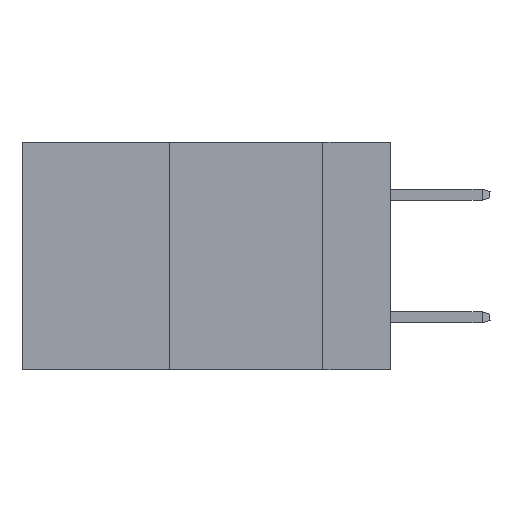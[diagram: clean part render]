
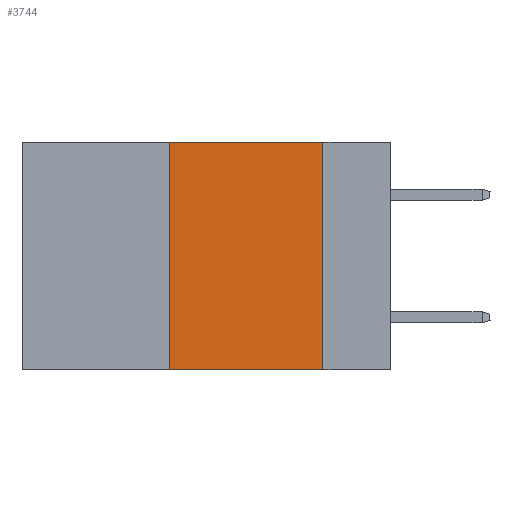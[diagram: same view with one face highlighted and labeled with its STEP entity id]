
A CAD part, left-side view. The second image highlights one B-rep face of the part: STEP entity #3744.
In plain terms, the highlighted planar face has unit normal (-1, 0, 0).
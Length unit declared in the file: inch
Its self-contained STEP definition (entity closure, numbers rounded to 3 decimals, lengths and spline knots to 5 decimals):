
#955 = CARTESIAN_POINT ( 'NONE',  ( 0., 0.11, 0. ) ) ;
#1171 = ORIENTED_EDGE ( 'NONE', *, *, #2881, .F. ) ;
#1340 = LINE ( 'NONE', #955, #3835 ) ;
#1670 = VERTEX_POINT ( 'NONE', #9632 ) ;
#1900 = ORIENTED_EDGE ( 'NONE', *, *, #5287, .T. ) ;
#2050 = VERTEX_POINT ( 'NONE', #5353 ) ;
#2430 = AXIS2_PLACEMENT_3D ( 'NONE', #10593, #5706, #5643 ) ;
#2775 = VERTEX_POINT ( 'NONE', #6938 ) ;
#2881 = EDGE_CURVE ( 'NONE', #2775, #2050, #11167, .T. ) ;
#3100 = DIRECTION ( 'NONE',  ( 0., 0., -1. ) ) ;
#3429 = ORIENTED_EDGE ( 'NONE', *, *, #8253, .F. ) ;
#3744 = ADVANCED_FACE ( 'NONE', ( #4328 ), #6311, .F. ) ;
#3835 = VECTOR ( 'NONE', #3100, 39.37008 ) ;
#4328 = FACE_OUTER_BOUND ( 'NONE', #7788, .T. ) ;
#5287 = EDGE_CURVE ( 'NONE', #2775, #1670, #8871, .T. ) ;
#5353 = CARTESIAN_POINT ( 'NONE',  ( 0., 0.36, 0. ) ) ;
#5643 = DIRECTION ( 'NONE',  ( 0., 0., -1. ) ) ;
#5706 = DIRECTION ( 'NONE',  ( 1., 0., 0. ) ) ;
#5998 = DIRECTION ( 'NONE',  ( 0., 0., 1. ) ) ;
#6028 = CARTESIAN_POINT ( 'NONE',  ( 0., 0.36, 0. ) ) ;
#6311 = PLANE ( 'NONE',  #2430 ) ;
#6621 = CARTESIAN_POINT ( 'NONE',  ( 0., 0.6, -0.37 ) ) ;
#6807 = EDGE_CURVE ( 'NONE', #9987, #1670, #1340, .T. ) ;
#6938 = CARTESIAN_POINT ( 'NONE',  ( 0., 0.36, -0.37 ) ) ;
#7747 = ORIENTED_EDGE ( 'NONE', *, *, #6807, .F. ) ;
#7788 = EDGE_LOOP ( 'NONE', ( #7747, #3429, #1171, #1900 ) ) ;
#8253 = EDGE_CURVE ( 'NONE', #2050, #9987, #12734, .T. ) ;
#8274 = VECTOR ( 'NONE', #12370, 39.37008 ) ;
#8312 = VECTOR ( 'NONE', #5998, 39.37008 ) ;
#8687 = CARTESIAN_POINT ( 'NONE',  ( 0., 0.11, 0. ) ) ;
#8871 = LINE ( 'NONE', #6621, #8274 ) ;
#9509 = CARTESIAN_POINT ( 'NONE',  ( 0., 0.6, 0. ) ) ;
#9553 = DIRECTION ( 'NONE',  ( 0., -1., 0. ) ) ;
#9632 = CARTESIAN_POINT ( 'NONE',  ( 0., 0.11, -0.37 ) ) ;
#9987 = VERTEX_POINT ( 'NONE', #8687 ) ;
#10225 = VECTOR ( 'NONE', #9553, 39.37008 ) ;
#10593 = CARTESIAN_POINT ( 'NONE',  ( 0., 0.6, 0. ) ) ;
#11167 = LINE ( 'NONE', #6028, #8312 ) ;
#12370 = DIRECTION ( 'NONE',  ( 0., -1., 0. ) ) ;
#12734 = LINE ( 'NONE', #9509, #10225 ) ;
